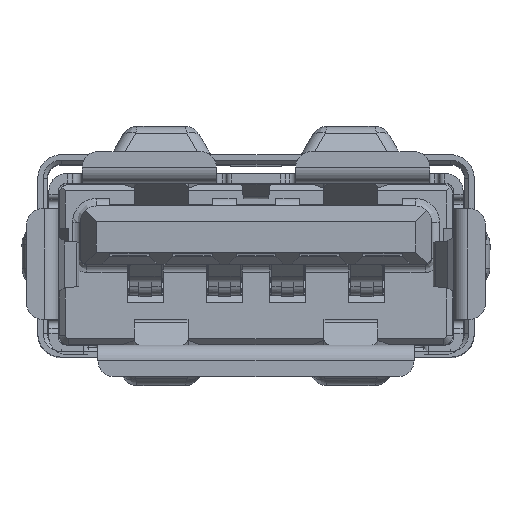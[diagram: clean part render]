
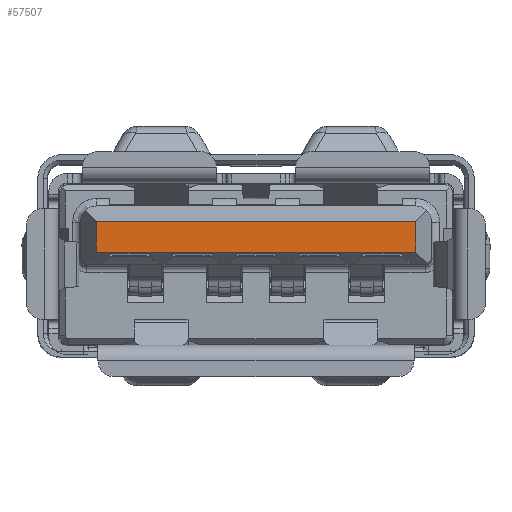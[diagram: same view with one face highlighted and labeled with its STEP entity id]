
A CAD part, top view. The second image highlights one B-rep face of the part: STEP entity #57507.
In plain terms, the highlighted face is planar.
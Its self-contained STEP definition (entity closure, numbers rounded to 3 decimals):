
#3510 = ORIENTED_EDGE ( 'NONE', *, *, #53285, .T. ) ;
#4424 = CARTESIAN_POINT ( 'NONE',  ( 5.05, -10.25, -1.34 ) ) ;
#4885 = VECTOR ( 'NONE', #67507, 1000. ) ;
#6949 = CARTESIAN_POINT ( 'NONE',  ( 5.252, -10.25, -0.355 ) ) ;
#7630 = DIRECTION ( 'NONE',  ( 0., -1., 0. ) ) ;
#9062 = VERTEX_POINT ( 'NONE', #4424 ) ;
#10919 = ORIENTED_EDGE ( 'NONE', *, *, #32000, .T. ) ;
#14042 = CARTESIAN_POINT ( 'NONE',  ( 0., -10.25, -1.34 ) ) ;
#14240 = LINE ( 'NONE', #61694, #4885 ) ;
#16898 = VECTOR ( 'NONE', #58943, 1000. ) ;
#23856 = AXIS2_PLACEMENT_3D ( 'NONE', #6949, #7630, #27783 ) ;
#24512 = CARTESIAN_POINT ( 'NONE',  ( -5.05, -10.25, -1.34 ) ) ;
#24971 = DIRECTION ( 'NONE',  ( 1., 0., 0. ) ) ;
#27783 = DIRECTION ( 'NONE',  ( -1., 0., 0. ) ) ;
#27859 = ORIENTED_EDGE ( 'NONE', *, *, #45264, .T. ) ;
#30586 = VERTEX_POINT ( 'NONE', #24512 ) ;
#30752 = LINE ( 'NONE', #14042, #46647 ) ;
#31815 = VERTEX_POINT ( 'NONE', #45348 ) ;
#32000 = EDGE_CURVE ( 'NONE', #31815, #30586, #49065, .T. ) ;
#32958 = LINE ( 'NONE', #58584, #16898 ) ;
#33901 = FACE_OUTER_BOUND ( 'NONE', #36351, .T. ) ;
#35963 = VECTOR ( 'NONE', #43947, 1000. ) ;
#36351 = EDGE_LOOP ( 'NONE', ( #3510, #10919, #27859, #39055 ) ) ;
#39055 = ORIENTED_EDGE ( 'NONE', *, *, #53466, .T. ) ;
#42817 = PLANE ( 'NONE',  #23856 ) ;
#43947 = DIRECTION ( 'NONE',  ( 0., 0., -1. ) ) ;
#44276 = CARTESIAN_POINT ( 'NONE',  ( -5.05, -10.25, -0.86 ) ) ;
#45264 = EDGE_CURVE ( 'NONE', #30586, #9062, #30752, .T. ) ;
#45348 = CARTESIAN_POINT ( 'NONE',  ( -5.05, -10.25, -0.38 ) ) ;
#46647 = VECTOR ( 'NONE', #24971, 1000. ) ;
#49065 = LINE ( 'NONE', #44276, #35963 ) ;
#49334 = VERTEX_POINT ( 'NONE', #49970 ) ;
#49970 = CARTESIAN_POINT ( 'NONE',  ( 5.05, -10.25, -0.38 ) ) ;
#53285 = EDGE_CURVE ( 'NONE', #49334, #31815, #14240, .T. ) ;
#53466 = EDGE_CURVE ( 'NONE', #9062, #49334, #32958, .T. ) ;
#57507 = ADVANCED_FACE ( 'NONE', ( #33901 ), #42817, .T. ) ;
#58584 = CARTESIAN_POINT ( 'NONE',  ( 5.05, -10.25, -0.86 ) ) ;
#58943 = DIRECTION ( 'NONE',  ( 0., 0., 1. ) ) ;
#61694 = CARTESIAN_POINT ( 'NONE',  ( 0., -10.25, -0.38 ) ) ;
#67507 = DIRECTION ( 'NONE',  ( -1., 0., 0. ) ) ;
